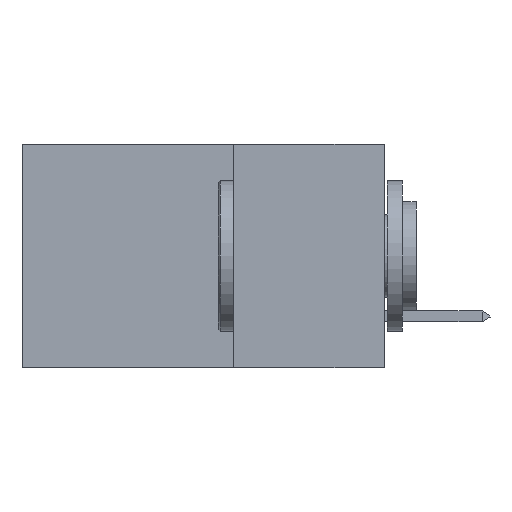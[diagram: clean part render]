
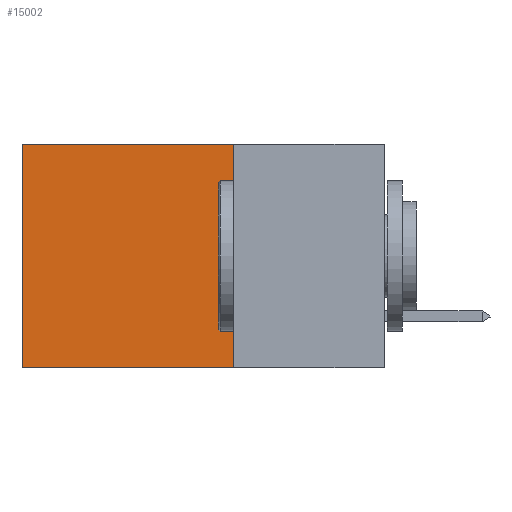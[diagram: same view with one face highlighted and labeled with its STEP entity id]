
A CAD part, left-side view. The second image highlights one B-rep face of the part: STEP entity #15002.
In plain terms, the highlighted planar face has unit normal (-1, 0, 0).
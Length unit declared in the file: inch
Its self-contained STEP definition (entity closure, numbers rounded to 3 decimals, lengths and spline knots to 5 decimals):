
#328 = EDGE_LOOP ( 'NONE', ( #33705, #31191, #8690, #29840 ) ) ;
#1000 = CARTESIAN_POINT ( 'NONE',  ( 0.2875, 0.25, -0.37 ) ) ;
#1119 = VERTEX_POINT ( 'NONE', #21502 ) ;
#2066 = CARTESIAN_POINT ( 'NONE',  ( 0.2875, 0.6, 0. ) ) ;
#2519 = EDGE_CURVE ( 'NONE', #11198, #20782, #19006, .T. ) ;
#5343 = CARTESIAN_POINT ( 'NONE',  ( 0.2875, 0.25, -0.37 ) ) ;
#7919 = CARTESIAN_POINT ( 'NONE',  ( 0.2875, 0.25, 0. ) ) ;
#8327 = VECTOR ( 'NONE', #10625, 39.37008 ) ;
#8690 = ORIENTED_EDGE ( 'NONE', *, *, #13485, .F. ) ;
#8843 = CARTESIAN_POINT ( 'NONE',  ( 0.2875, 0.25, 0. ) ) ;
#10598 = PLANE ( 'NONE',  #16297 ) ;
#10625 = DIRECTION ( 'NONE',  ( 0., 1., 0. ) ) ;
#11198 = VERTEX_POINT ( 'NONE', #7919 ) ;
#11462 = CARTESIAN_POINT ( 'NONE',  ( 0.2875, 0.25, 0. ) ) ;
#12356 = DIRECTION ( 'NONE',  ( 0., 1., 0. ) ) ;
#13485 = EDGE_CURVE ( 'NONE', #11198, #34745, #25080, .T. ) ;
#15002 = ADVANCED_FACE ( 'NONE', ( #15084 ), #10598, .F. ) ;
#15084 = FACE_OUTER_BOUND ( 'NONE', #328, .T. ) ;
#16297 = AXIS2_PLACEMENT_3D ( 'NONE', #11462, #18055, #31013 ) ;
#16557 = VECTOR ( 'NONE', #20032, 39.37008 ) ;
#17614 = CARTESIAN_POINT ( 'NONE',  ( 0.2875, 0.6, 0. ) ) ;
#18055 = DIRECTION ( 'NONE',  ( 1., 0., 0. ) ) ;
#19006 = LINE ( 'NONE', #8843, #21488 ) ;
#20032 = DIRECTION ( 'NONE',  ( 0., 0., -1. ) ) ;
#20782 = VERTEX_POINT ( 'NONE', #2066 ) ;
#21488 = VECTOR ( 'NONE', #12356, 39.37008 ) ;
#21502 = CARTESIAN_POINT ( 'NONE',  ( 0.2875, 0.6, -0.37 ) ) ;
#22287 = EDGE_CURVE ( 'NONE', #20782, #1119, #27255, .T. ) ;
#25080 = LINE ( 'NONE', #29223, #16557 ) ;
#27255 = LINE ( 'NONE', #17614, #35363 ) ;
#29223 = CARTESIAN_POINT ( 'NONE',  ( 0.2875, 0.25, 0. ) ) ;
#29840 = ORIENTED_EDGE ( 'NONE', *, *, #2519, .T. ) ;
#31013 = DIRECTION ( 'NONE',  ( 0., 0., -1. ) ) ;
#31191 = ORIENTED_EDGE ( 'NONE', *, *, #34544, .F. ) ;
#33705 = ORIENTED_EDGE ( 'NONE', *, *, #22287, .T. ) ;
#33820 = DIRECTION ( 'NONE',  ( 0., 0., -1. ) ) ;
#34544 = EDGE_CURVE ( 'NONE', #34745, #1119, #38430, .T. ) ;
#34745 = VERTEX_POINT ( 'NONE', #5343 ) ;
#35363 = VECTOR ( 'NONE', #33820, 39.37008 ) ;
#38430 = LINE ( 'NONE', #1000, #8327 ) ;
